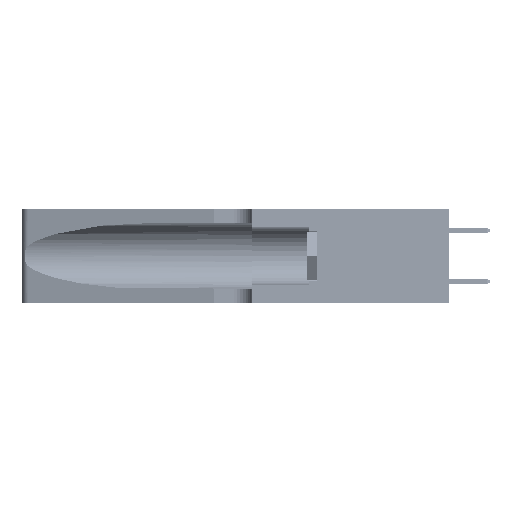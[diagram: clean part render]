
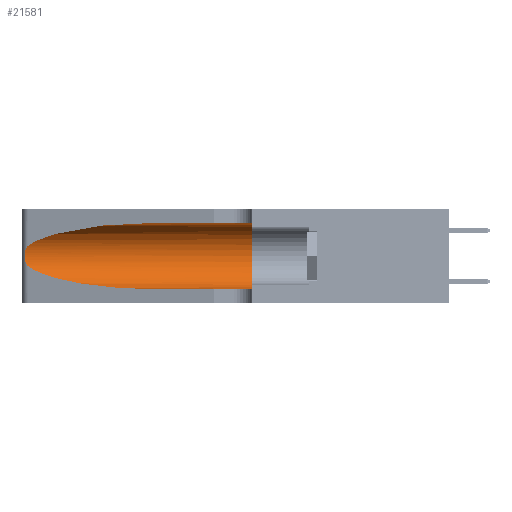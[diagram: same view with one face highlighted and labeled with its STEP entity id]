
A CAD part, left-side view. The second image highlights one B-rep face of the part: STEP entity #21581.
In plain terms, the highlighted cylindrical face has radius 3.308 mm (diameter 6.617 mm), a partial arc.
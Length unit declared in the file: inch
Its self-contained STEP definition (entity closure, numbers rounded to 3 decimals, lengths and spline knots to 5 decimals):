
#6 = EDGE_CURVE ( 'NONE', #17172, #18031, #27953, .T. ) ;
#3331 = CARTESIAN_POINT ( 'NONE',  ( 0.26075, 1.23896, 0.178 ) ) ;
#3600 = CARTESIAN_POINT ( 'NONE',  ( 0.25487, 1.22718, 0.22369 ) ) ;
#3741 = DIRECTION ( 'NONE',  ( 0., -1., 0. ) ) ;
#3797 = FACE_OUTER_BOUND ( 'NONE', #6465, .T. ) ;
#3930 = LINE ( 'NONE', #19758, #43669 ) ;
#4264 = CARTESIAN_POINT ( 'NONE',  ( 0.1305, 1.61858, 0.185 ) ) ;
#6465 = EDGE_LOOP ( 'NONE', ( #49051, #48792, #32827, #16584, #32362, #43755 ) ) ;
#7576 = CARTESIAN_POINT ( 'NONE',  ( 0.25639, 1.23184, 0.21858 ) ) ;
#7622 = B_SPLINE_CURVE_WITH_KNOTS ( 'NONE', 3,
 ( #31190, #51311, #7576, #11453, #47597, #39609, #44035, #3331, #39432, #39793, #15515, #51472, #19730, #31522 ),
 .UNSPECIFIED., .F., .F.,
 ( 4, 2, 2, 2, 2, 2, 4 ),
 ( 0., 0.00027, 0.00053, 0.00107, 0.0016, 0.00187, 0.00214 ),
 .UNSPECIFIED. ) ;
#7910 = DIRECTION ( 'NONE',  ( 0., 0., 1. ) ) ;
#11453 = CARTESIAN_POINT ( 'NONE',  ( 0.25787, 1.23484, 0.2124 ) ) ;
#11771 = CARTESIAN_POINT ( 'NONE',  ( 0.1305, 0.35, 0.185 ) ) ;
#12821 = EDGE_CURVE ( 'NONE', #25529, #16075, #42515, .T. ) ;
#14400 = AXIS2_PLACEMENT_3D ( 'NONE', #11771, #35743, #7910 ) ;
#15515 = CARTESIAN_POINT ( 'NONE',  ( 0.25789, 1.23486, 0.15765 ) ) ;
#16075 = VERTEX_POINT ( 'NONE', #16815 ) ;
#16584 = ORIENTED_EDGE ( 'NONE', *, *, #12821, .T. ) ;
#16815 = CARTESIAN_POINT ( 'NONE',  ( 0.1305, 0.35, 0.05475 ) ) ;
#17172 = VERTEX_POINT ( 'NONE', #25076 ) ;
#18031 = VERTEX_POINT ( 'NONE', #38520 ) ;
#18346 = DIRECTION ( 'NONE',  ( 0., -1., 0. ) ) ;
#19275 = EDGE_CURVE ( 'NONE', #47169, #25529, #26369, .T. ) ;
#19730 = CARTESIAN_POINT ( 'NONE',  ( 0.25555, 1.22993, 0.14849 ) ) ;
#19758 = CARTESIAN_POINT ( 'NONE',  ( 0.1305, 1.61858, 0.31525 ) ) ;
#21581 = ADVANCED_FACE ( 'NONE', ( #3797 ), #51761, .F. ) ;
#23530 = CARTESIAN_POINT ( 'NONE',  ( 0.2373, 1.15595, 0.28018 ) ) ;
#24859 = VECTOR ( 'NONE', #18346, 39.37008 ) ;
#25076 = CARTESIAN_POINT ( 'NONE',  ( 0.1305, 0.72297, 0.31525 ) ) ;
#25529 = VERTEX_POINT ( 'NONE', #48493 ) ;
#25557 = EDGE_CURVE ( 'NONE', #17172, #36748, #3930, .T. ) ;
#26369 =( BOUNDED_CURVE ( )  B_SPLINE_CURVE ( 3, ( #34908, #47258, #42131, #50117 ),
 .UNSPECIFIED., .F., .T. ) 
 B_SPLINE_CURVE_WITH_KNOTS ( ( 4, 4 ),
 ( 3.44316, 4.71239 ),
 .UNSPECIFIED. ) 
 CURVE ( )  GEOMETRIC_REPRESENTATION_ITEM ( )  RATIONAL_B_SPLINE_CURVE ( ( 1., 0.87, 0.87, 1. ) ) 
 REPRESENTATION_ITEM ( '' )  );
#27470 = CARTESIAN_POINT ( 'NONE',  ( 0.1305, 0.35, 0.31525 ) ) ;
#27953 =( BOUNDED_CURVE ( )  B_SPLINE_CURVE ( 3, ( #39532, #43964, #23530, #3600 ),
 .UNSPECIFIED., .F., .F. ) 
 B_SPLINE_CURVE_WITH_KNOTS ( ( 4, 4 ),
 ( 1.5708, 2.84003 ),
 .UNSPECIFIED. ) 
 CURVE ( )  GEOMETRIC_REPRESENTATION_ITEM ( )  RATIONAL_B_SPLINE_CURVE ( ( 1., 0.87, 0.87, 1. ) ) 
 REPRESENTATION_ITEM ( '' )  );
#31190 = CARTESIAN_POINT ( 'NONE',  ( 0.25487, 1.22718, 0.22369 ) ) ;
#31522 = CARTESIAN_POINT ( 'NONE',  ( 0.25487, 1.22718, 0.14631 ) ) ;
#32362 = ORIENTED_EDGE ( 'NONE', *, *, #32788, .F. ) ;
#32788 = EDGE_CURVE ( 'NONE', #36748, #16075, #45564, .T. ) ;
#32827 = ORIENTED_EDGE ( 'NONE', *, *, #19275, .T. ) ;
#34908 = CARTESIAN_POINT ( 'NONE',  ( 0.25487, 1.22718, 0.14631 ) ) ;
#35743 = DIRECTION ( 'NONE',  ( 0., 1., 0. ) ) ;
#36027 = EDGE_CURVE ( 'NONE', #18031, #47169, #7622, .T. ) ;
#36748 = VERTEX_POINT ( 'NONE', #27470 ) ;
#36976 = AXIS2_PLACEMENT_3D ( 'NONE', #4264, #3741, #52228 ) ;
#38520 = CARTESIAN_POINT ( 'NONE',  ( 0.25487, 1.22718, 0.22369 ) ) ;
#39432 = CARTESIAN_POINT ( 'NONE',  ( 0.26017, 1.23833, 0.17102 ) ) ;
#39532 = CARTESIAN_POINT ( 'NONE',  ( 0.1305, 0.72297, 0.31525 ) ) ;
#39609 = CARTESIAN_POINT ( 'NONE',  ( 0.26018, 1.23835, 0.19895 ) ) ;
#39793 = CARTESIAN_POINT ( 'NONE',  ( 0.25856, 1.23593, 0.16098 ) ) ;
#42131 = CARTESIAN_POINT ( 'NONE',  ( 0.18966, 0.96281, 0.05475 ) ) ;
#42515 = LINE ( 'NONE', #43007, #24859 ) ;
#43007 = CARTESIAN_POINT ( 'NONE',  ( 0.1305, 1.61858, 0.05475 ) ) ;
#43669 = VECTOR ( 'NONE', #44235, 39.37008 ) ;
#43755 = ORIENTED_EDGE ( 'NONE', *, *, #25557, .F. ) ;
#43964 = CARTESIAN_POINT ( 'NONE',  ( 0.18966, 0.96281, 0.31525 ) ) ;
#44035 = CARTESIAN_POINT ( 'NONE',  ( 0.26075, 1.23896, 0.19203 ) ) ;
#44235 = DIRECTION ( 'NONE',  ( 0., -1., 0. ) ) ;
#45564 = CIRCLE ( 'NONE', #14400, 0.13025 ) ;
#47169 = VERTEX_POINT ( 'NONE', #51328 ) ;
#47258 = CARTESIAN_POINT ( 'NONE',  ( 0.2373, 1.15595, 0.08982 ) ) ;
#47597 = CARTESIAN_POINT ( 'NONE',  ( 0.25854, 1.2359, 0.20912 ) ) ;
#48493 = CARTESIAN_POINT ( 'NONE',  ( 0.1305, 0.72297, 0.05475 ) ) ;
#48792 = ORIENTED_EDGE ( 'NONE', *, *, #36027, .T. ) ;
#49051 = ORIENTED_EDGE ( 'NONE', *, *, #6, .T. ) ;
#50117 = CARTESIAN_POINT ( 'NONE',  ( 0.1305, 0.72297, 0.05475 ) ) ;
#51311 = CARTESIAN_POINT ( 'NONE',  ( 0.25555, 1.22994, 0.2215 ) ) ;
#51328 = CARTESIAN_POINT ( 'NONE',  ( 0.25487, 1.22718, 0.14631 ) ) ;
#51472 = CARTESIAN_POINT ( 'NONE',  ( 0.25639, 1.23186, 0.15144 ) ) ;
#51761 = CYLINDRICAL_SURFACE ( 'NONE', #36976, 0.13025 ) ;
#52228 = DIRECTION ( 'NONE',  ( 0., 0., -1. ) ) ;
